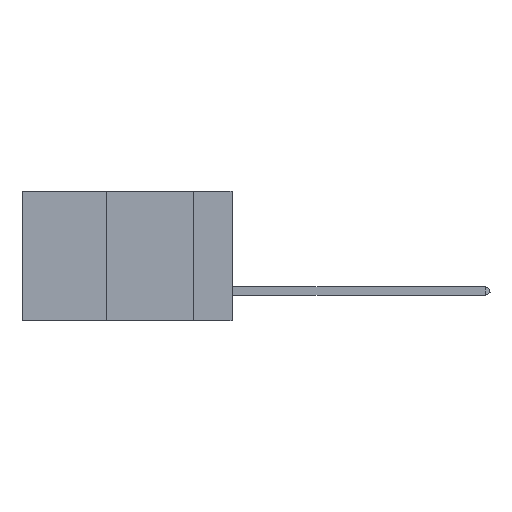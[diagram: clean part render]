
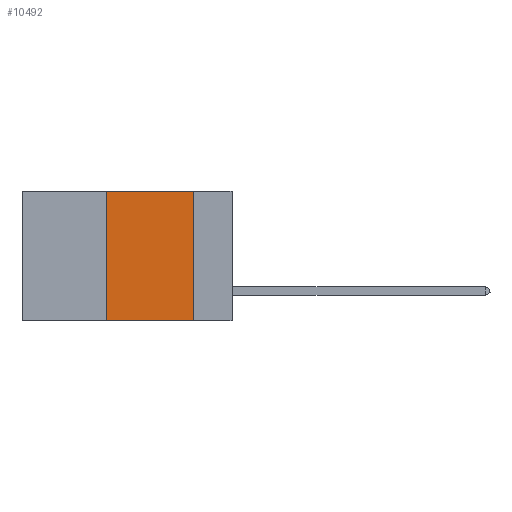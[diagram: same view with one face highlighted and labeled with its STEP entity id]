
A CAD part, left-side view. The second image highlights one B-rep face of the part: STEP entity #10492.
In plain terms, the highlighted planar face has unit normal (-1, 0, 0).
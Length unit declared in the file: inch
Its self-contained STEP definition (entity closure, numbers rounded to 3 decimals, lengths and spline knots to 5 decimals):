
#237 = VERTEX_POINT ( 'NONE', #14894 ) ;
#600 = DIRECTION ( 'NONE',  ( 0., -1., 0. ) ) ;
#1675 = CARTESIAN_POINT ( 'NONE',  ( 0., 0.11, 0. ) ) ;
#1750 = CARTESIAN_POINT ( 'NONE',  ( 0., 0.36, 0. ) ) ;
#2708 = CARTESIAN_POINT ( 'NONE',  ( 0., 0.11, 0. ) ) ;
#3958 = EDGE_CURVE ( 'NONE', #12386, #237, #15110, .T. ) ;
#4836 = CARTESIAN_POINT ( 'NONE',  ( 0., 0.6, 0. ) ) ;
#7026 = LINE ( 'NONE', #15084, #15232 ) ;
#7668 = CARTESIAN_POINT ( 'NONE',  ( 0., 0.6, -0.37 ) ) ;
#7747 = DIRECTION ( 'NONE',  ( 0., 0., -1. ) ) ;
#8482 = CARTESIAN_POINT ( 'NONE',  ( 0., 0.36, -0.37 ) ) ;
#8971 = DIRECTION ( 'NONE',  ( 0., 0., -1. ) ) ;
#10368 = VECTOR ( 'NONE', #8971, 39.37008 ) ;
#10492 = ADVANCED_FACE ( 'NONE', ( #11340 ), #12670, .F. ) ;
#11340 = FACE_OUTER_BOUND ( 'NONE', #18332, .T. ) ;
#11484 = EDGE_CURVE ( 'NONE', #18079, #17677, #14052, .T. ) ;
#11577 = CARTESIAN_POINT ( 'NONE',  ( 0., 0.36, 0. ) ) ;
#12050 = VECTOR ( 'NONE', #14517, 39.37008 ) ;
#12386 = VERTEX_POINT ( 'NONE', #1675 ) ;
#12670 = PLANE ( 'NONE',  #19031 ) ;
#12801 = VECTOR ( 'NONE', #17114, 39.37008 ) ;
#13840 = ORIENTED_EDGE ( 'NONE', *, *, #11484, .F. ) ;
#14052 = LINE ( 'NONE', #1750, #12050 ) ;
#14127 = DIRECTION ( 'NONE',  ( 1., 0., 0. ) ) ;
#14517 = DIRECTION ( 'NONE',  ( 0., 0., 1. ) ) ;
#14894 = CARTESIAN_POINT ( 'NONE',  ( 0., 0.11, -0.37 ) ) ;
#15084 = CARTESIAN_POINT ( 'NONE',  ( 0., 0.6, 0. ) ) ;
#15110 = LINE ( 'NONE', #2708, #10368 ) ;
#15232 = VECTOR ( 'NONE', #600, 39.37008 ) ;
#16786 = EDGE_CURVE ( 'NONE', #18079, #237, #18251, .T. ) ;
#16817 = ORIENTED_EDGE ( 'NONE', *, *, #19902, .F. ) ;
#17114 = DIRECTION ( 'NONE',  ( 0., -1., 0. ) ) ;
#17677 = VERTEX_POINT ( 'NONE', #11577 ) ;
#17900 = ORIENTED_EDGE ( 'NONE', *, *, #16786, .T. ) ;
#18079 = VERTEX_POINT ( 'NONE', #8482 ) ;
#18251 = LINE ( 'NONE', #7668, #12801 ) ;
#18332 = EDGE_LOOP ( 'NONE', ( #20416, #16817, #13840, #17900 ) ) ;
#19031 = AXIS2_PLACEMENT_3D ( 'NONE', #4836, #14127, #7747 ) ;
#19902 = EDGE_CURVE ( 'NONE', #17677, #12386, #7026, .T. ) ;
#20416 = ORIENTED_EDGE ( 'NONE', *, *, #3958, .F. ) ;
